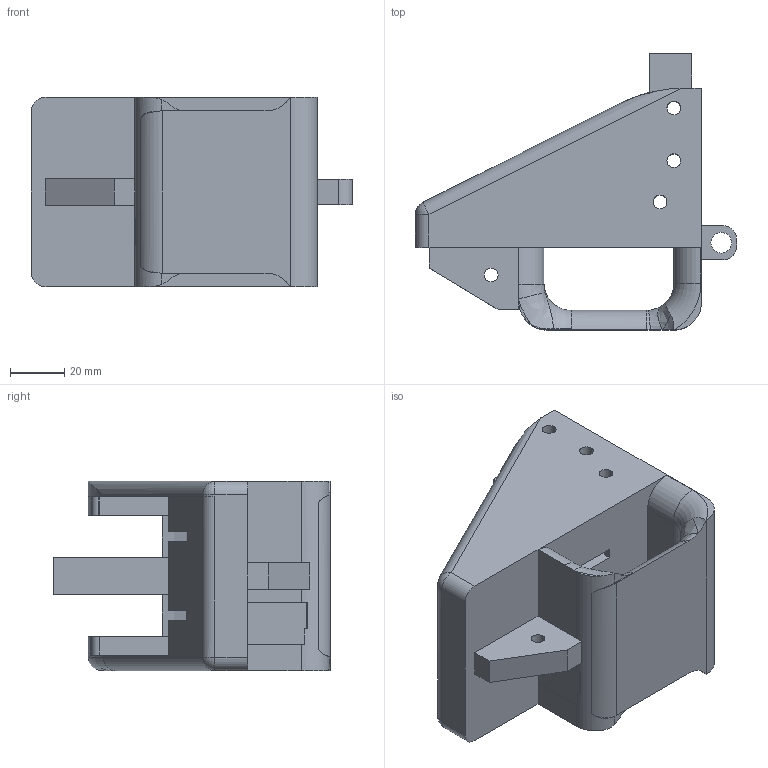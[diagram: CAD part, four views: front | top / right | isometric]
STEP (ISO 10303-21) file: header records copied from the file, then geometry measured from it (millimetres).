
FILE_DESCRIPTION (( 'STEP AP214' ), '1' );
FILE_NAME ('410receiver.STEP', '2013-07-25T16:57:31', ( '' ), ( '' ), 'SwSTEP 2.0', 'SolidWorks 2013', '' );
FILE_SCHEMA (( 'AUTOMOTIVE_DESIGN' ));
Length unit declared in the file: millimetre
Products named in the file (1): 410receiver
Bounding box: 118.54 x 102.01 x 69.85 mm (x, y, z)
Volume: 204440.5 mm3; surface area: 58794.4 mm2
Topology: 1 solids, 1 shells, 163 faces, 460 edges, 296 vertices
Faces by surface type: plane 89, cylinder 57, bspline 10, torus 5, sphere 2
Entity records: 5855 total; most frequent: CARTESIAN_POINT 1541, ORIENTED_EDGE 920, DIRECTION 867, EDGE_CURVE 460, VERTEX_POINT 296, LINE 295, VECTOR 295, AXIS2_PLACEMENT_3D 286
